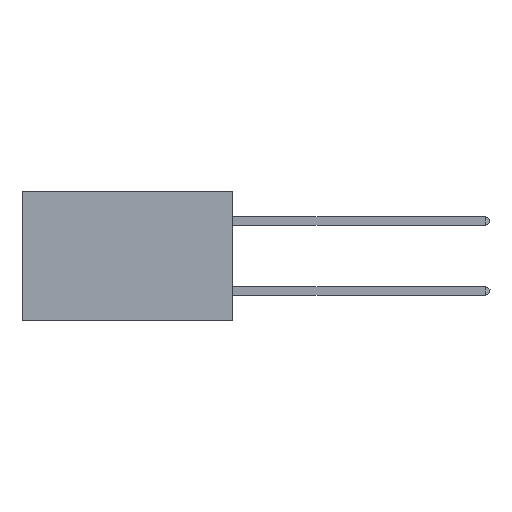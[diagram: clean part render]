
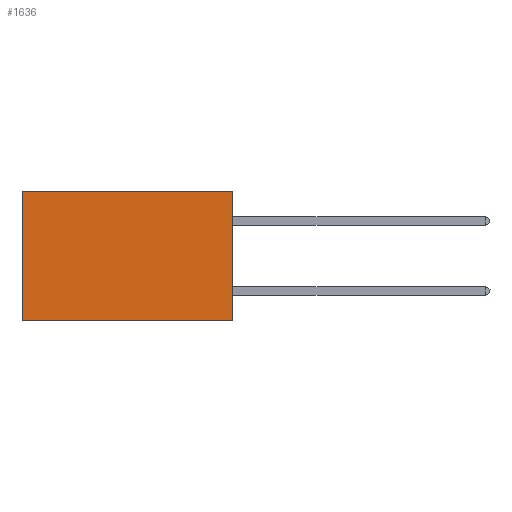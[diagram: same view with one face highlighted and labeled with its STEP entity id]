
A CAD part, left-side view. The second image highlights one B-rep face of the part: STEP entity #1636.
In plain terms, the highlighted planar face has unit normal (-1, 0, 0).
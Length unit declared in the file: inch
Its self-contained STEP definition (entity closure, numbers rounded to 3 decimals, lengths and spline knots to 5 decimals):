
#167 = VECTOR ( 'NONE', #6492, 39.37008 ) ;
#394 = DIRECTION ( 'NONE',  ( 0., 1., 0. ) ) ;
#1491 = DIRECTION ( 'NONE',  ( 0., 0., -1. ) ) ;
#1636 = ADVANCED_FACE ( 'NONE', ( #13009 ), #2999, .F. ) ;
#1960 = DIRECTION ( 'NONE',  ( 1., 0., 0. ) ) ;
#2080 = CARTESIAN_POINT ( 'NONE',  ( 0.2875, 0., 0. ) ) ;
#2383 = VECTOR ( 'NONE', #1491, 39.37008 ) ;
#2736 = CARTESIAN_POINT ( 'NONE',  ( 0.2875, 0., 0. ) ) ;
#2781 = LINE ( 'NONE', #2080, #11234 ) ;
#2820 = ORIENTED_EDGE ( 'NONE', *, *, #5987, .F. ) ;
#2999 = PLANE ( 'NONE',  #10464 ) ;
#3310 = VERTEX_POINT ( 'NONE', #9034 ) ;
#3548 = VECTOR ( 'NONE', #394, 39.37008 ) ;
#3627 = LINE ( 'NONE', #2736, #167 ) ;
#4600 = VERTEX_POINT ( 'NONE', #5777 ) ;
#5155 = EDGE_CURVE ( 'NONE', #4600, #9394, #2781, .T. ) ;
#5777 = CARTESIAN_POINT ( 'NONE',  ( 0.2875, 0., 0. ) ) ;
#5947 = CARTESIAN_POINT ( 'NONE',  ( 0.2875, 0.6, 0. ) ) ;
#5987 = EDGE_CURVE ( 'NONE', #4600, #3310, #3627, .T. ) ;
#6198 = LINE ( 'NONE', #5947, #2383 ) ;
#6492 = DIRECTION ( 'NONE',  ( 0., 0., -1. ) ) ;
#6650 = CARTESIAN_POINT ( 'NONE',  ( 0.2875, 0.6, -0.37 ) ) ;
#6777 = CARTESIAN_POINT ( 'NONE',  ( 0.2875, 0.6, 0. ) ) ;
#7515 = CARTESIAN_POINT ( 'NONE',  ( 0.2875, 0., 0. ) ) ;
#7754 = LINE ( 'NONE', #12712, #3548 ) ;
#8447 = EDGE_LOOP ( 'NONE', ( #13024, #11081, #2820, #9064 ) ) ;
#8630 = DIRECTION ( 'NONE',  ( 0., 0., -1. ) ) ;
#8938 = VERTEX_POINT ( 'NONE', #6650 ) ;
#9034 = CARTESIAN_POINT ( 'NONE',  ( 0.2875, 0., -0.37 ) ) ;
#9064 = ORIENTED_EDGE ( 'NONE', *, *, #5155, .T. ) ;
#9394 = VERTEX_POINT ( 'NONE', #6777 ) ;
#9425 = EDGE_CURVE ( 'NONE', #3310, #8938, #7754, .T. ) ;
#10197 = DIRECTION ( 'NONE',  ( 0., 1., 0. ) ) ;
#10464 = AXIS2_PLACEMENT_3D ( 'NONE', #7515, #1960, #8630 ) ;
#11081 = ORIENTED_EDGE ( 'NONE', *, *, #9425, .F. ) ;
#11234 = VECTOR ( 'NONE', #10197, 39.37008 ) ;
#12712 = CARTESIAN_POINT ( 'NONE',  ( 0.2875, 0., -0.37 ) ) ;
#13009 = FACE_OUTER_BOUND ( 'NONE', #8447, .T. ) ;
#13024 = ORIENTED_EDGE ( 'NONE', *, *, #13441, .T. ) ;
#13441 = EDGE_CURVE ( 'NONE', #9394, #8938, #6198, .T. ) ;
